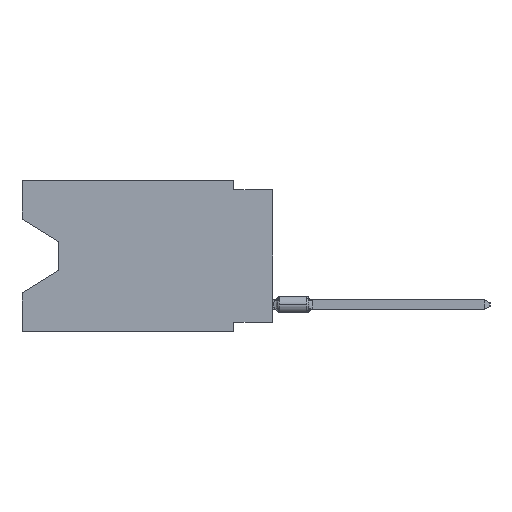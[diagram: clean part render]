
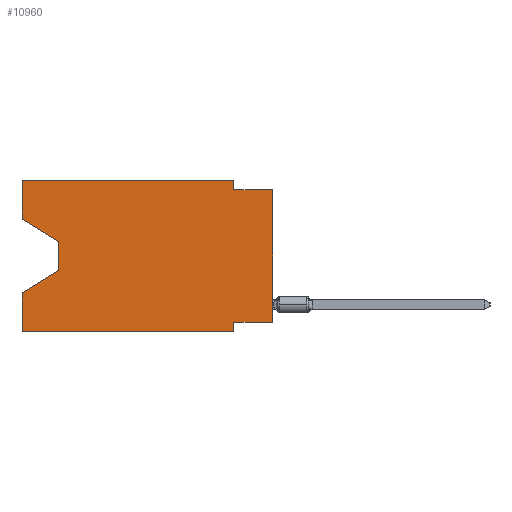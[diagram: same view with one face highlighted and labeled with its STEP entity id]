
A CAD part, left-side view. The second image highlights one B-rep face of the part: STEP entity #10960.
In plain terms, the highlighted planar face has unit normal (-1, 0, 0).
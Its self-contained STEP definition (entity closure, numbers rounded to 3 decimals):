
#758 = VECTOR ( 'NONE', #21971, 1000. ) ;
#1909 = EDGE_CURVE ( 'NONE', #66732, #27597, #50026, .T. ) ;
#6573 = EDGE_LOOP ( 'NONE', ( #51588, #29360, #12620, #32132, #57421, #69832, #16444, #49231, #11424, #72660, #27121, #64590 ) ) ;
#7896 = VECTOR ( 'NONE', #19466, 1000. ) ;
#8456 = VECTOR ( 'NONE', #25565, 1000. ) ;
#8577 = VERTEX_POINT ( 'NONE', #24121 ) ;
#8976 = EDGE_CURVE ( 'NONE', #66732, #8577, #61861, .T. ) ;
#9652 = VERTEX_POINT ( 'NONE', #54999 ) ;
#9720 = DIRECTION ( 'NONE',  ( 0., -1., 0. ) ) ;
#10960 = ADVANCED_FACE ( 'NONE', ( #53478 ), #66615, .F. ) ;
#10982 = CARTESIAN_POINT ( 'NONE',  ( 0., 0., 0. ) ) ;
#11424 = ORIENTED_EDGE ( 'NONE', *, *, #28461, .F. ) ;
#11729 = VERTEX_POINT ( 'NONE', #78400 ) ;
#12620 = ORIENTED_EDGE ( 'NONE', *, *, #33589, .T. ) ;
#13052 = CARTESIAN_POINT ( 'NONE',  ( 0., 2.54, -0.635 ) ) ;
#13725 = CARTESIAN_POINT ( 'NONE',  ( 0., 16.383, -9.906 ) ) ;
#14199 = VERTEX_POINT ( 'NONE', #53350 ) ;
#14468 = LINE ( 'NONE', #44884, #8456 ) ;
#16020 = EDGE_CURVE ( 'NONE', #41511, #9652, #64355, .T. ) ;
#16290 = LINE ( 'NONE', #72615, #31801 ) ;
#16444 = ORIENTED_EDGE ( 'NONE', *, *, #77345, .F. ) ;
#19466 = DIRECTION ( 'NONE',  ( 0., 0., -1. ) ) ;
#19555 = VECTOR ( 'NONE', #9720, 1000. ) ;
#19949 = EDGE_CURVE ( 'NONE', #9652, #41405, #73034, .T. ) ;
#21177 = CARTESIAN_POINT ( 'NONE',  ( 0., 13.97, -4.013 ) ) ;
#21971 = DIRECTION ( 'NONE',  ( 0., 0.855, -0.519 ) ) ;
#23389 = CARTESIAN_POINT ( 'NONE',  ( 0., 16.383, -2.546 ) ) ;
#24121 = CARTESIAN_POINT ( 'NONE',  ( 0., 16.383, -7.36 ) ) ;
#25565 = DIRECTION ( 'NONE',  ( 0., -0.855, -0.519 ) ) ;
#27121 = ORIENTED_EDGE ( 'NONE', *, *, #19949, .F. ) ;
#27597 = VERTEX_POINT ( 'NONE', #46915 ) ;
#28461 = EDGE_CURVE ( 'NONE', #45314, #11729, #16290, .T. ) ;
#29360 = ORIENTED_EDGE ( 'NONE', *, *, #71723, .T. ) ;
#31801 = VECTOR ( 'NONE', #49152, 1000. ) ;
#32132 = ORIENTED_EDGE ( 'NONE', *, *, #8976, .F. ) ;
#33589 = EDGE_CURVE ( 'NONE', #75431, #8577, #59791, .T. ) ;
#33912 = VECTOR ( 'NONE', #61942, 1000. ) ;
#34697 = DIRECTION ( 'NONE',  ( 0., 0., 1. ) ) ;
#35228 = LINE ( 'NONE', #10982, #33912 ) ;
#37971 = CARTESIAN_POINT ( 'NONE',  ( 0., 2.54, -9.906 ) ) ;
#38374 = EDGE_CURVE ( 'NONE', #58821, #11729, #35228, .T. ) ;
#40451 = VECTOR ( 'NONE', #80228, 1000. ) ;
#41405 = VERTEX_POINT ( 'NONE', #80904 ) ;
#41511 = VERTEX_POINT ( 'NONE', #23389 ) ;
#43028 = CARTESIAN_POINT ( 'NONE',  ( 0., 2.54, -9.271 ) ) ;
#43459 = DIRECTION ( 'NONE',  ( 0., -1., 0. ) ) ;
#44884 = CARTESIAN_POINT ( 'NONE',  ( 0., 16.383, -2.546 ) ) ;
#44904 = CARTESIAN_POINT ( 'NONE',  ( 0., 0., -9.271 ) ) ;
#45314 = VERTEX_POINT ( 'NONE', #13052 ) ;
#46233 = DIRECTION ( 'NONE',  ( 0., 0., -1. ) ) ;
#46915 = CARTESIAN_POINT ( 'NONE',  ( 0., 2.54, -9.906 ) ) ;
#47035 = CARTESIAN_POINT ( 'NONE',  ( 0., 13.97, -5.893 ) ) ;
#48054 = CARTESIAN_POINT ( 'NONE',  ( 0., 13.97, -5.893 ) ) ;
#48529 = EDGE_CURVE ( 'NONE', #41405, #45314, #55568, .T. ) ;
#49152 = DIRECTION ( 'NONE',  ( 0., -1., 0. ) ) ;
#49231 = ORIENTED_EDGE ( 'NONE', *, *, #38374, .T. ) ;
#50026 = LINE ( 'NONE', #50831, #79633 ) ;
#50831 = CARTESIAN_POINT ( 'NONE',  ( 0., 16.383, -9.906 ) ) ;
#51588 = ORIENTED_EDGE ( 'NONE', *, *, #56563, .T. ) ;
#52119 = EDGE_CURVE ( 'NONE', #66187, #27597, #63447, .T. ) ;
#53213 = LINE ( 'NONE', #21177, #54516 ) ;
#53350 = CARTESIAN_POINT ( 'NONE',  ( 0., 13.97, -4.013 ) ) ;
#53478 = FACE_OUTER_BOUND ( 'NONE', #6573, .T. ) ;
#54491 = DIRECTION ( 'NONE',  ( 0., 1., 0. ) ) ;
#54516 = VECTOR ( 'NONE', #46233, 1000. ) ;
#54999 = CARTESIAN_POINT ( 'NONE',  ( 0., 16.383, 0. ) ) ;
#55173 = CARTESIAN_POINT ( 'NONE',  ( 0., 2.54, 0. ) ) ;
#55568 = LINE ( 'NONE', #55173, #40451 ) ;
#56498 = CARTESIAN_POINT ( 'NONE',  ( 0., 16.383, 0. ) ) ;
#56563 = EDGE_CURVE ( 'NONE', #41511, #14199, #14468, .T. ) ;
#57421 = ORIENTED_EDGE ( 'NONE', *, *, #1909, .T. ) ;
#58174 = CARTESIAN_POINT ( 'NONE',  ( 0., 16.383, 0. ) ) ;
#58821 = VERTEX_POINT ( 'NONE', #44904 ) ;
#59208 = VECTOR ( 'NONE', #69224, 1000. ) ;
#59640 = DIRECTION ( 'NONE',  ( 1., 0., 0. ) ) ;
#59791 = LINE ( 'NONE', #47035, #758 ) ;
#61861 = LINE ( 'NONE', #56498, #59208 ) ;
#61942 = DIRECTION ( 'NONE',  ( 0., 0., 1. ) ) ;
#63447 = LINE ( 'NONE', #37971, #7896 ) ;
#64355 = LINE ( 'NONE', #58174, #65950 ) ;
#64590 = ORIENTED_EDGE ( 'NONE', *, *, #16020, .F. ) ;
#65821 = DIRECTION ( 'NONE',  ( 0., 0., -1. ) ) ;
#65950 = VECTOR ( 'NONE', #34697, 1000. ) ;
#66040 = CARTESIAN_POINT ( 'NONE',  ( 0., 16.383, 0. ) ) ;
#66187 = VERTEX_POINT ( 'NONE', #43028 ) ;
#66615 = PLANE ( 'NONE',  #75722 ) ;
#66732 = VERTEX_POINT ( 'NONE', #13725 ) ;
#66825 = CARTESIAN_POINT ( 'NONE',  ( 0., 0., -9.271 ) ) ;
#69224 = DIRECTION ( 'NONE',  ( 0., 0., 1. ) ) ;
#69832 = ORIENTED_EDGE ( 'NONE', *, *, #52119, .F. ) ;
#71578 = CARTESIAN_POINT ( 'NONE',  ( 0., 16.383, 0. ) ) ;
#71723 = EDGE_CURVE ( 'NONE', #14199, #75431, #53213, .T. ) ;
#72615 = CARTESIAN_POINT ( 'NONE',  ( 0., 0., -0.635 ) ) ;
#72660 = ORIENTED_EDGE ( 'NONE', *, *, #48529, .F. ) ;
#73034 = LINE ( 'NONE', #66040, #19555 ) ;
#74281 = VECTOR ( 'NONE', #54491, 1000. ) ;
#75431 = VERTEX_POINT ( 'NONE', #48054 ) ;
#75722 = AXIS2_PLACEMENT_3D ( 'NONE', #71578, #59640, #65821 ) ;
#77345 = EDGE_CURVE ( 'NONE', #58821, #66187, #79973, .T. ) ;
#78400 = CARTESIAN_POINT ( 'NONE',  ( 0., 0., -0.635 ) ) ;
#79633 = VECTOR ( 'NONE', #43459, 1000. ) ;
#79973 = LINE ( 'NONE', #66825, #74281 ) ;
#80228 = DIRECTION ( 'NONE',  ( 0., 0., -1. ) ) ;
#80904 = CARTESIAN_POINT ( 'NONE',  ( 0., 2.54, 0. ) ) ;
